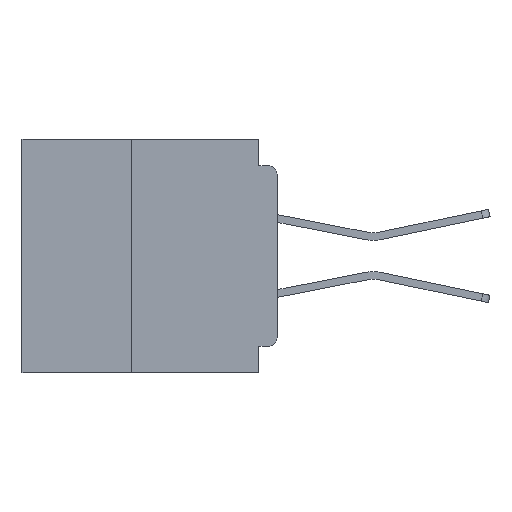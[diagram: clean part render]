
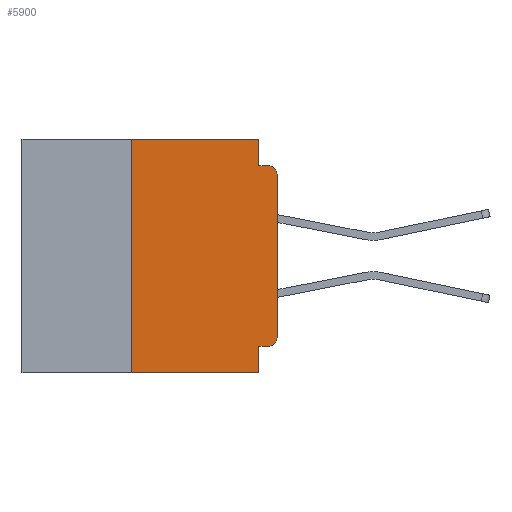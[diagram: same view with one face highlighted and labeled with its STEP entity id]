
A CAD part, left-side view. The second image highlights one B-rep face of the part: STEP entity #5900.
In plain terms, the highlighted planar face has unit normal (-1, 0, 0).
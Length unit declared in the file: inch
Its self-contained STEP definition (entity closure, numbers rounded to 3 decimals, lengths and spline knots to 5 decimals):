
#338 = CIRCLE ( 'NONE', #11366, 0.015 ) ;
#1496 = CARTESIAN_POINT ( 'NONE',  ( 0., 0.437, 0. ) ) ;
#2169 = VERTEX_POINT ( 'NONE', #37919 ) ;
#2172 = LINE ( 'NONE', #32557, #17243 ) ;
#2368 = LINE ( 'NONE', #27797, #26166 ) ;
#4329 = DIRECTION ( 'NONE',  ( 0., 0., -1. ) ) ;
#4404 = LINE ( 'NONE', #34200, #10576 ) ;
#4552 = DIRECTION ( 'NONE',  ( 0., -1., 0. ) ) ;
#4710 = LINE ( 'NONE', #33342, #36252 ) ;
#4776 = VERTEX_POINT ( 'NONE', #9243 ) ;
#4854 = EDGE_LOOP ( 'NONE', ( #18672, #18740, #19858, #19900, #20904, #21006, #21585, #21655, #21947, #22214 ) ) ;
#5030 = DIRECTION ( 'NONE',  ( 0., 0., -1. ) ) ;
#5035 = DIRECTION ( 'NONE',  ( 1., 0., 0. ) ) ;
#5127 = PLANE ( 'NONE',  #10131 ) ;
#5594 = CARTESIAN_POINT ( 'NONE',  ( 0., 0.437, 0. ) ) ;
#5631 = CARTESIAN_POINT ( 'NONE',  ( 0., 0.25, 0. ) ) ;
#5900 = ADVANCED_FACE ( 'NONE', ( #19700 ), #5127, .F. ) ;
#6223 = EDGE_CURVE ( 'NONE', #22365, #29202, #338, .T. ) ;
#6922 = LINE ( 'NONE', #21375, #21858 ) ;
#8443 = CARTESIAN_POINT ( 'NONE',  ( 0., 0.015, -0.045 ) ) ;
#9010 = VERTEX_POINT ( 'NONE', #5631 ) ;
#9243 = CARTESIAN_POINT ( 'NONE',  ( 0., 0.031, -0.045 ) ) ;
#9524 = DIRECTION ( 'NONE',  ( 0., 1., 0. ) ) ;
#9836 = VERTEX_POINT ( 'NONE', #13053 ) ;
#10131 = AXIS2_PLACEMENT_3D ( 'NONE', #5594, #5035, #5030 ) ;
#10145 = EDGE_CURVE ( 'NONE', #20427, #9010, #19892, .T. ) ;
#10562 = CARTESIAN_POINT ( 'NONE',  ( 0., 0.031, 0. ) ) ;
#10576 = VECTOR ( 'NONE', #13577, 39.37008 ) ;
#11361 = CARTESIAN_POINT ( 'NONE',  ( 0., 0.25, -0.4 ) ) ;
#11366 = AXIS2_PLACEMENT_3D ( 'NONE', #16689, #16479, #16568 ) ;
#11496 = DIRECTION ( 'NONE',  ( 0., 0., 1. ) ) ;
#11695 = CARTESIAN_POINT ( 'NONE',  ( 0., 0.015, -0.355 ) ) ;
#12336 = EDGE_CURVE ( 'NONE', #9836, #17880, #2368, .T. ) ;
#12665 = AXIS2_PLACEMENT_3D ( 'NONE', #33007, #15334, #35951 ) ;
#13053 = CARTESIAN_POINT ( 'NONE',  ( 0., 0.031, -0.355 ) ) ;
#13577 = DIRECTION ( 'NONE',  ( 0., -1., 0. ) ) ;
#14057 = CARTESIAN_POINT ( 'NONE',  ( 0., 0., -0.34 ) ) ;
#14138 = EDGE_CURVE ( 'NONE', #9010, #2169, #26796, .T. ) ;
#14504 = VECTOR ( 'NONE', #4329, 39.37008 ) ;
#14795 = EDGE_CURVE ( 'NONE', #4776, #28020, #4404, .T. ) ;
#14976 = CIRCLE ( 'NONE', #12665, 0.015 ) ;
#15334 = DIRECTION ( 'NONE',  ( -1., 0., 0. ) ) ;
#15694 = DIRECTION ( 'NONE',  ( 0., -1., 0. ) ) ;
#16479 = DIRECTION ( 'NONE',  ( -1., 0., 0. ) ) ;
#16568 = DIRECTION ( 'NONE',  ( 0., 0., -1. ) ) ;
#16689 = CARTESIAN_POINT ( 'NONE',  ( 0., 0.015, -0.34 ) ) ;
#17243 = VECTOR ( 'NONE', #23601, 39.37008 ) ;
#17880 = VERTEX_POINT ( 'NONE', #30940 ) ;
#18672 = ORIENTED_EDGE ( 'NONE', *, *, #34893, .T. ) ;
#18740 = ORIENTED_EDGE ( 'NONE', *, *, #25883, .T. ) ;
#19036 = VECTOR ( 'NONE', #4552, 39.37008 ) ;
#19700 = FACE_OUTER_BOUND ( 'NONE', #4854, .T. ) ;
#19858 = ORIENTED_EDGE ( 'NONE', *, *, #14795, .F. ) ;
#19892 = LINE ( 'NONE', #11361, #34566 ) ;
#19900 = ORIENTED_EDGE ( 'NONE', *, *, #22114, .F. ) ;
#20427 = VERTEX_POINT ( 'NONE', #36141 ) ;
#20904 = ORIENTED_EDGE ( 'NONE', *, *, #14138, .F. ) ;
#21006 = ORIENTED_EDGE ( 'NONE', *, *, #10145, .F. ) ;
#21375 = CARTESIAN_POINT ( 'NONE',  ( 0., 0., -0.355 ) ) ;
#21585 = ORIENTED_EDGE ( 'NONE', *, *, #31412, .T. ) ;
#21655 = ORIENTED_EDGE ( 'NONE', *, *, #12336, .F. ) ;
#21858 = VECTOR ( 'NONE', #9524, 39.37008 ) ;
#21947 = ORIENTED_EDGE ( 'NONE', *, *, #27615, .F. ) ;
#22114 = EDGE_CURVE ( 'NONE', #2169, #4776, #22469, .T. ) ;
#22214 = ORIENTED_EDGE ( 'NONE', *, *, #6223, .T. ) ;
#22365 = VERTEX_POINT ( 'NONE', #11695 ) ;
#22469 = LINE ( 'NONE', #10562, #14504 ) ;
#23601 = DIRECTION ( 'NONE',  ( 0., 0., 1. ) ) ;
#25826 = CARTESIAN_POINT ( 'NONE',  ( 0., 0., -0.06 ) ) ;
#25883 = EDGE_CURVE ( 'NONE', #32365, #28020, #14976, .T. ) ;
#26166 = VECTOR ( 'NONE', #36526, 39.37008 ) ;
#26796 = LINE ( 'NONE', #1496, #19036 ) ;
#27615 = EDGE_CURVE ( 'NONE', #22365, #9836, #6922, .T. ) ;
#27797 = CARTESIAN_POINT ( 'NONE',  ( 0., 0.031, -0.4 ) ) ;
#28020 = VERTEX_POINT ( 'NONE', #8443 ) ;
#29202 = VERTEX_POINT ( 'NONE', #14057 ) ;
#30940 = CARTESIAN_POINT ( 'NONE',  ( 0., 0.031, -0.4 ) ) ;
#31412 = EDGE_CURVE ( 'NONE', #20427, #17880, #4710, .T. ) ;
#32365 = VERTEX_POINT ( 'NONE', #25826 ) ;
#32557 = CARTESIAN_POINT ( 'NONE',  ( 0., 0., 0. ) ) ;
#33007 = CARTESIAN_POINT ( 'NONE',  ( 0., 0.015, -0.06 ) ) ;
#33342 = CARTESIAN_POINT ( 'NONE',  ( 0., 0.437, -0.4 ) ) ;
#34200 = CARTESIAN_POINT ( 'NONE',  ( 0., 0., -0.045 ) ) ;
#34566 = VECTOR ( 'NONE', #11496, 39.37008 ) ;
#34893 = EDGE_CURVE ( 'NONE', #29202, #32365, #2172, .T. ) ;
#35951 = DIRECTION ( 'NONE',  ( 0., 0., -1. ) ) ;
#36141 = CARTESIAN_POINT ( 'NONE',  ( 0., 0.25, -0.4 ) ) ;
#36252 = VECTOR ( 'NONE', #15694, 39.37008 ) ;
#36526 = DIRECTION ( 'NONE',  ( 0., 0., -1. ) ) ;
#37919 = CARTESIAN_POINT ( 'NONE',  ( 0., 0.031, 0. ) ) ;
